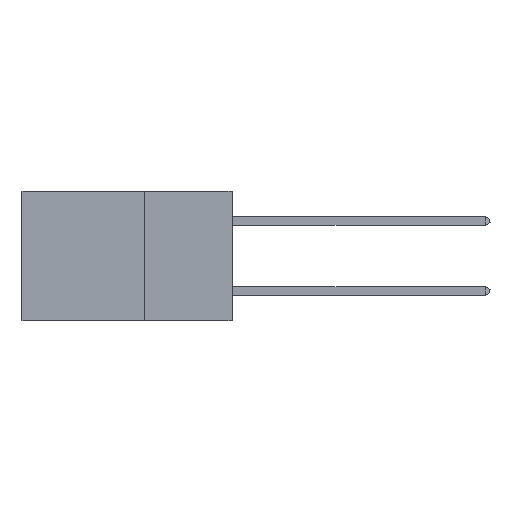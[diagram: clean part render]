
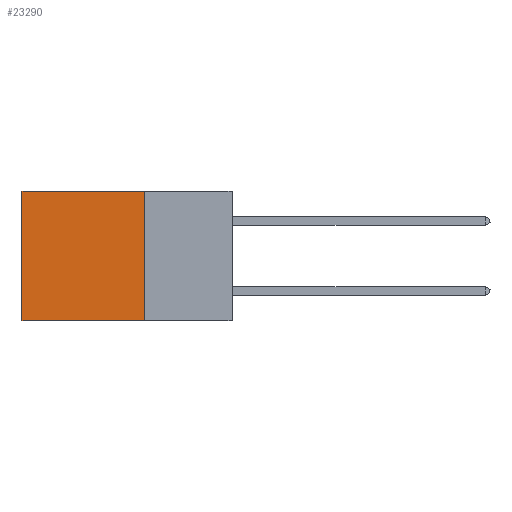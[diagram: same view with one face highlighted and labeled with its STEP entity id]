
A CAD part, left-side view. The second image highlights one B-rep face of the part: STEP entity #23290.
In plain terms, the highlighted planar face has unit normal (-1, 0, 0).
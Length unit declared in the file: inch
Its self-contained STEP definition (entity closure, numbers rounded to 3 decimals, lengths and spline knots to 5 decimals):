
#589 = VERTEX_POINT ( 'NONE', #23904 ) ;
#4476 = CARTESIAN_POINT ( 'NONE',  ( 0.2875, 0.25, -0.37 ) ) ;
#5682 = EDGE_CURVE ( 'NONE', #589, #38244, #29557, .T. ) ;
#7402 = CARTESIAN_POINT ( 'NONE',  ( 0.2875, 0.6, 0. ) ) ;
#7415 = EDGE_LOOP ( 'NONE', ( #30457, #29465, #33323, #37612 ) ) ;
#8160 = LINE ( 'NONE', #7402, #23643 ) ;
#10215 = VECTOR ( 'NONE', #27759, 39.37008 ) ;
#11391 = VECTOR ( 'NONE', #23032, 39.37008 ) ;
#12401 = LINE ( 'NONE', #16849, #11391 ) ;
#13652 = DIRECTION ( 'NONE',  ( 0., 0., -1. ) ) ;
#16849 = CARTESIAN_POINT ( 'NONE',  ( 0.2875, 0.25, -0.37 ) ) ;
#16933 = DIRECTION ( 'NONE',  ( 0., 0., -1. ) ) ;
#18503 = LINE ( 'NONE', #21642, #10215 ) ;
#19188 = EDGE_CURVE ( 'NONE', #30046, #35687, #8160, .T. ) ;
#20026 = CARTESIAN_POINT ( 'NONE',  ( 0.2875, 0.6, -0.37 ) ) ;
#21045 = AXIS2_PLACEMENT_3D ( 'NONE', #30637, #39747, #21579 ) ;
#21579 = DIRECTION ( 'NONE',  ( 0., 0., -1. ) ) ;
#21642 = CARTESIAN_POINT ( 'NONE',  ( 0.2875, 0.25, 0. ) ) ;
#23032 = DIRECTION ( 'NONE',  ( 0., 1., 0. ) ) ;
#23290 = ADVANCED_FACE ( 'NONE', ( #25229 ), #36589, .F. ) ;
#23643 = VECTOR ( 'NONE', #13652, 39.37008 ) ;
#23904 = CARTESIAN_POINT ( 'NONE',  ( 0.2875, 0.25, 0. ) ) ;
#25229 = FACE_OUTER_BOUND ( 'NONE', #7415, .T. ) ;
#27759 = DIRECTION ( 'NONE',  ( 0., 1., 0. ) ) ;
#29465 = ORIENTED_EDGE ( 'NONE', *, *, #35010, .F. ) ;
#29557 = LINE ( 'NONE', #32142, #37616 ) ;
#30046 = VERTEX_POINT ( 'NONE', #39547 ) ;
#30457 = ORIENTED_EDGE ( 'NONE', *, *, #19188, .T. ) ;
#30637 = CARTESIAN_POINT ( 'NONE',  ( 0.2875, 0.25, 0. ) ) ;
#32142 = CARTESIAN_POINT ( 'NONE',  ( 0.2875, 0.25, 0. ) ) ;
#33323 = ORIENTED_EDGE ( 'NONE', *, *, #5682, .F. ) ;
#35010 = EDGE_CURVE ( 'NONE', #38244, #35687, #12401, .T. ) ;
#35687 = VERTEX_POINT ( 'NONE', #20026 ) ;
#36589 = PLANE ( 'NONE',  #21045 ) ;
#37612 = ORIENTED_EDGE ( 'NONE', *, *, #39470, .T. ) ;
#37616 = VECTOR ( 'NONE', #16933, 39.37008 ) ;
#38244 = VERTEX_POINT ( 'NONE', #4476 ) ;
#39470 = EDGE_CURVE ( 'NONE', #589, #30046, #18503, .T. ) ;
#39547 = CARTESIAN_POINT ( 'NONE',  ( 0.2875, 0.6, 0. ) ) ;
#39747 = DIRECTION ( 'NONE',  ( 1., 0., 0. ) ) ;
